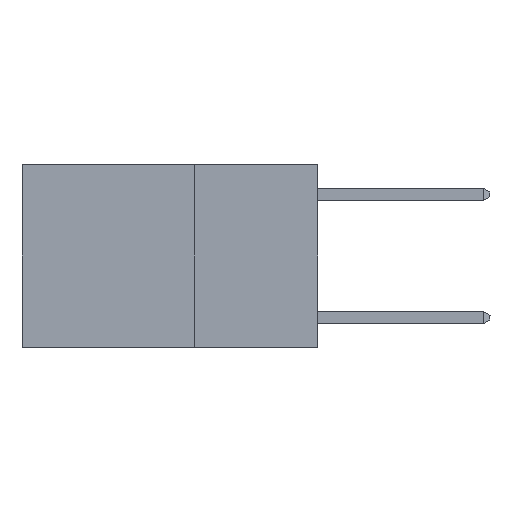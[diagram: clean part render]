
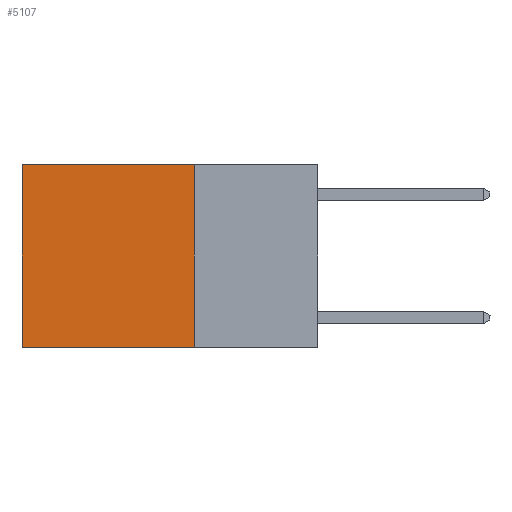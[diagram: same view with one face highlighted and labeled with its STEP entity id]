
A CAD part, left-side view. The second image highlights one B-rep face of the part: STEP entity #5107.
In plain terms, the highlighted planar face has unit normal (-1, 0, 0).
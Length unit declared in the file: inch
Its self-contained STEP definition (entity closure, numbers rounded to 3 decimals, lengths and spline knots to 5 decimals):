
#610 = VERTEX_POINT ( 'NONE', #6135 ) ;
#755 = VECTOR ( 'NONE', #13634, 39.37008 ) ;
#1411 = DIRECTION ( 'NONE',  ( 0., 0., -1. ) ) ;
#1708 = CARTESIAN_POINT ( 'NONE',  ( 0.2625, 0.25, 0. ) ) ;
#2463 = CARTESIAN_POINT ( 'NONE',  ( 0.2625, 0.25, 0. ) ) ;
#2800 = DIRECTION ( 'NONE',  ( 0., 0., -1. ) ) ;
#3163 = ORIENTED_EDGE ( 'NONE', *, *, #6318, .F. ) ;
#3556 = DIRECTION ( 'NONE',  ( 0., 1., 0. ) ) ;
#3782 = EDGE_CURVE ( 'NONE', #8437, #10706, #8692, .T. ) ;
#3856 = ORIENTED_EDGE ( 'NONE', *, *, #3782, .T. ) ;
#3993 = LINE ( 'NONE', #10535, #755 ) ;
#4573 = VECTOR ( 'NONE', #13081, 39.37008 ) ;
#4662 = CARTESIAN_POINT ( 'NONE',  ( 0.2625, 0.25, 0. ) ) ;
#4718 = ORIENTED_EDGE ( 'NONE', *, *, #9405, .T. ) ;
#5107 = ADVANCED_FACE ( 'NONE', ( #7979 ), #13252, .F. ) ;
#5555 = LINE ( 'NONE', #1708, #8133 ) ;
#6135 = CARTESIAN_POINT ( 'NONE',  ( 0.2625, 0.25, -0.37 ) ) ;
#6318 = EDGE_CURVE ( 'NONE', #8437, #610, #5555, .T. ) ;
#7534 = LINE ( 'NONE', #12051, #4573 ) ;
#7979 = FACE_OUTER_BOUND ( 'NONE', #8983, .T. ) ;
#8005 = DIRECTION ( 'NONE',  ( 1., 0., 0. ) ) ;
#8133 = VECTOR ( 'NONE', #2800, 39.37008 ) ;
#8437 = VERTEX_POINT ( 'NONE', #12786 ) ;
#8692 = LINE ( 'NONE', #2463, #10864 ) ;
#8983 = EDGE_LOOP ( 'NONE', ( #4718, #10523, #3163, #3856 ) ) ;
#9405 = EDGE_CURVE ( 'NONE', #10706, #10771, #7534, .T. ) ;
#9439 = CARTESIAN_POINT ( 'NONE',  ( 0.2625, 0.6, -0.37 ) ) ;
#9459 = AXIS2_PLACEMENT_3D ( 'NONE', #4662, #8005, #1411 ) ;
#10523 = ORIENTED_EDGE ( 'NONE', *, *, #11543, .F. ) ;
#10535 = CARTESIAN_POINT ( 'NONE',  ( 0.2625, 0.25, -0.37 ) ) ;
#10706 = VERTEX_POINT ( 'NONE', #12119 ) ;
#10771 = VERTEX_POINT ( 'NONE', #9439 ) ;
#10864 = VECTOR ( 'NONE', #3556, 39.37008 ) ;
#11543 = EDGE_CURVE ( 'NONE', #610, #10771, #3993, .T. ) ;
#12051 = CARTESIAN_POINT ( 'NONE',  ( 0.2625, 0.6, 0. ) ) ;
#12119 = CARTESIAN_POINT ( 'NONE',  ( 0.2625, 0.6, 0. ) ) ;
#12786 = CARTESIAN_POINT ( 'NONE',  ( 0.2625, 0.25, 0. ) ) ;
#13081 = DIRECTION ( 'NONE',  ( 0., 0., -1. ) ) ;
#13252 = PLANE ( 'NONE',  #9459 ) ;
#13634 = DIRECTION ( 'NONE',  ( 0., 1., 0. ) ) ;
